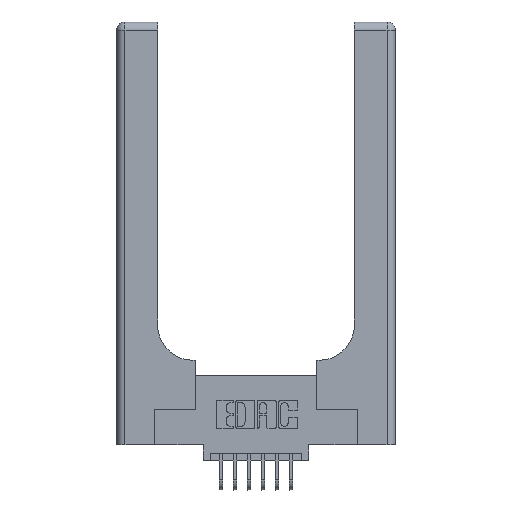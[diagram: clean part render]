
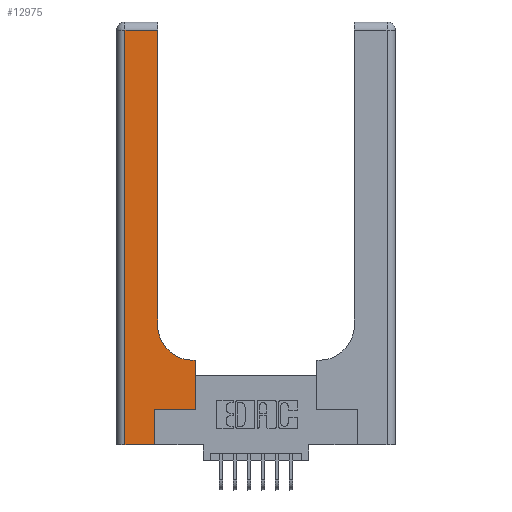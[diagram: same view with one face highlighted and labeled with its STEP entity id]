
A CAD part, top view. The second image highlights one B-rep face of the part: STEP entity #12975.
In plain terms, the highlighted planar face has unit normal (0, 0, 1).
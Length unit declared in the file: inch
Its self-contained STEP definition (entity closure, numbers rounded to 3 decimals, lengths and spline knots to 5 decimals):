
#128 = DIRECTION ( 'NONE',  ( 1., 0., 0. ) ) ;
#894 = DIRECTION ( 'NONE',  ( -1., 0., 0. ) ) ;
#905 = ORIENTED_EDGE ( 'NONE', *, *, #8691, .T. ) ;
#1467 = CARTESIAN_POINT ( 'NONE',  ( 0.5585, 0.6, 0.37 ) ) ;
#1674 = LINE ( 'NONE', #15006, #3251 ) ;
#1692 = CARTESIAN_POINT ( 'NONE',  ( 0.2915, 0.85, 0.37 ) ) ;
#1895 = VECTOR ( 'NONE', #16523, 39.37008 ) ;
#1930 = AXIS2_PLACEMENT_3D ( 'NONE', #10190, #8911, #12665 ) ;
#2228 = CARTESIAN_POINT ( 'NONE',  ( 0.06, 0., 0.37 ) ) ;
#2408 = CARTESIAN_POINT ( 'NONE',  ( 0., 0., 0.37 ) ) ;
#2793 = DIRECTION ( 'NONE',  ( 0., 0., -1. ) ) ;
#2922 = EDGE_CURVE ( 'NONE', #9948, #12084, #7304, .T. ) ;
#3165 = EDGE_CURVE ( 'NONE', #14237, #4009, #15316, .T. ) ;
#3251 = VECTOR ( 'NONE', #7390, 39.37008 ) ;
#3404 = CARTESIAN_POINT ( 'NONE',  ( 0.2915, 3., 0.37 ) ) ;
#3473 = DIRECTION ( 'NONE',  ( 0., 1., 0. ) ) ;
#4009 = VERTEX_POINT ( 'NONE', #8327 ) ;
#4644 = DIRECTION ( 'NONE',  ( 0., 1., 0. ) ) ;
#5423 = EDGE_CURVE ( 'NONE', #7205, #14237, #12641, .T. ) ;
#6266 = EDGE_CURVE ( 'NONE', #9770, #7205, #1674, .T. ) ;
#6304 = CARTESIAN_POINT ( 'NONE',  ( 0.5585, 0.25, 0.37 ) ) ;
#6351 = DIRECTION ( 'NONE',  ( 0., -1., 0. ) ) ;
#6988 = VECTOR ( 'NONE', #15119, 39.37008 ) ;
#7205 = VERTEX_POINT ( 'NONE', #6304 ) ;
#7304 = LINE ( 'NONE', #15323, #8693 ) ;
#7390 = DIRECTION ( 'NONE',  ( 1., 0., 0. ) ) ;
#7622 = LINE ( 'NONE', #3404, #9611 ) ;
#7821 = EDGE_CURVE ( 'NONE', #11933, #13100, #7622, .T. ) ;
#7957 = CARTESIAN_POINT ( 'NONE',  ( 0.5415, 0.85, 0.37 ) ) ;
#8327 = CARTESIAN_POINT ( 'NONE',  ( 0.5415, 0.6, 0.37 ) ) ;
#8560 = CARTESIAN_POINT ( 'NONE',  ( 0., 2.94, 0.37 ) ) ;
#8691 = EDGE_CURVE ( 'NONE', #13100, #9948, #10774, .T. ) ;
#8693 = VECTOR ( 'NONE', #6351, 39.37008 ) ;
#8762 = VERTEX_POINT ( 'NONE', #8998 ) ;
#8911 = DIRECTION ( 'NONE',  ( 0., 0., -1. ) ) ;
#8998 = CARTESIAN_POINT ( 'NONE',  ( 0.269, 0., 0.37 ) ) ;
#9556 = DIRECTION ( 'NONE',  ( 0., 1., 0. ) ) ;
#9592 = ORIENTED_EDGE ( 'NONE', *, *, #15506, .T. ) ;
#9611 = VECTOR ( 'NONE', #4644, 39.37008 ) ;
#9770 = VERTEX_POINT ( 'NONE', #13986 ) ;
#9914 = ORIENTED_EDGE ( 'NONE', *, *, #10608, .T. ) ;
#9948 = VERTEX_POINT ( 'NONE', #12271 ) ;
#10190 = CARTESIAN_POINT ( 'NONE',  ( 0., 3., 0.37 ) ) ;
#10356 = CARTESIAN_POINT ( 'NONE',  ( 0.2915, 2.94, 0.37 ) ) ;
#10608 = EDGE_CURVE ( 'NONE', #4009, #11933, #12727, .T. ) ;
#10669 = VECTOR ( 'NONE', #894, 39.37008 ) ;
#10774 = LINE ( 'NONE', #8560, #6988 ) ;
#11222 = ORIENTED_EDGE ( 'NONE', *, *, #5423, .T. ) ;
#11495 = VECTOR ( 'NONE', #3473, 39.37008 ) ;
#11933 = VERTEX_POINT ( 'NONE', #1692 ) ;
#12084 = VERTEX_POINT ( 'NONE', #2228 ) ;
#12239 = ORIENTED_EDGE ( 'NONE', *, *, #7821, .T. ) ;
#12271 = CARTESIAN_POINT ( 'NONE',  ( 0.06, 2.94, 0.37 ) ) ;
#12301 = CARTESIAN_POINT ( 'NONE',  ( 0.269, 0., 0.37 ) ) ;
#12303 = ORIENTED_EDGE ( 'NONE', *, *, #3165, .T. ) ;
#12418 = CARTESIAN_POINT ( 'NONE',  ( 0.2915, 0.6, 0.37 ) ) ;
#12488 = EDGE_LOOP ( 'NONE', ( #12239, #905, #15664, #9592, #13492, #14242, #11222, #12303, #9914 ) ) ;
#12641 = LINE ( 'NONE', #13158, #15857 ) ;
#12665 = DIRECTION ( 'NONE',  ( -1., 0., 0. ) ) ;
#12723 = PLANE ( 'NONE',  #1930 ) ;
#12727 = CIRCLE ( 'NONE', #13886, 0.25 ) ;
#12975 = ADVANCED_FACE ( 'NONE', ( #14356 ), #12723, .F. ) ;
#13100 = VERTEX_POINT ( 'NONE', #10356 ) ;
#13158 = CARTESIAN_POINT ( 'NONE',  ( 0.5585, 0.25, 0.37 ) ) ;
#13288 = LINE ( 'NONE', #2408, #1895 ) ;
#13492 = ORIENTED_EDGE ( 'NONE', *, *, #15299, .T. ) ;
#13886 = AXIS2_PLACEMENT_3D ( 'NONE', #7957, #2793, #128 ) ;
#13986 = CARTESIAN_POINT ( 'NONE',  ( 0.269, 0.25, 0.37 ) ) ;
#14105 = LINE ( 'NONE', #12301, #11495 ) ;
#14237 = VERTEX_POINT ( 'NONE', #1467 ) ;
#14242 = ORIENTED_EDGE ( 'NONE', *, *, #6266, .T. ) ;
#14356 = FACE_OUTER_BOUND ( 'NONE', #12488, .T. ) ;
#15006 = CARTESIAN_POINT ( 'NONE',  ( 0.269, 0.25, 0.37 ) ) ;
#15119 = DIRECTION ( 'NONE',  ( -1., 0., 0. ) ) ;
#15299 = EDGE_CURVE ( 'NONE', #8762, #9770, #14105, .T. ) ;
#15316 = LINE ( 'NONE', #12418, #10669 ) ;
#15323 = CARTESIAN_POINT ( 'NONE',  ( 0.06, 3., 0.37 ) ) ;
#15506 = EDGE_CURVE ( 'NONE', #12084, #8762, #13288, .T. ) ;
#15664 = ORIENTED_EDGE ( 'NONE', *, *, #2922, .T. ) ;
#15857 = VECTOR ( 'NONE', #9556, 39.37008 ) ;
#16523 = DIRECTION ( 'NONE',  ( 1., 0., 0. ) ) ;
